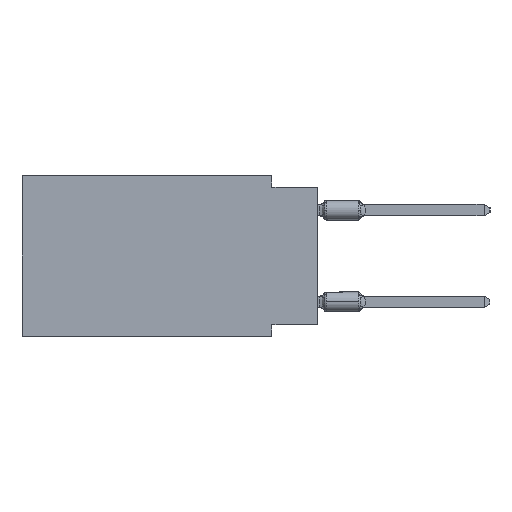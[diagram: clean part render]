
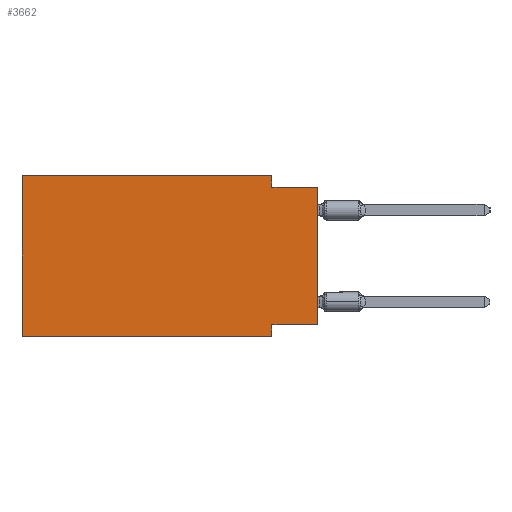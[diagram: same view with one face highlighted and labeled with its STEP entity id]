
A CAD part, left-side view. The second image highlights one B-rep face of the part: STEP entity #3662.
In plain terms, the highlighted planar face has unit normal (-1, 0, 0).
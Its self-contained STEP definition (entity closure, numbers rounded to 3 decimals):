
#502 = ORIENTED_EDGE ( 'NONE', *, *, #22959, .F. ) ;
#1128 = VERTEX_POINT ( 'NONE', #4056 ) ;
#3191 = VERTEX_POINT ( 'NONE', #32529 ) ;
#3344 = ORIENTED_EDGE ( 'NONE', *, *, #11986, .F. ) ;
#3662 = ADVANCED_FACE ( 'NONE', ( #44472 ), #28444, .F. ) ;
#3699 = EDGE_CURVE ( 'NONE', #20973, #11544, #36913, .T. ) ;
#3856 = ORIENTED_EDGE ( 'NONE', *, *, #19612, .F. ) ;
#4056 = CARTESIAN_POINT ( 'NONE',  ( 0., 16.383, 0. ) ) ;
#4516 = LINE ( 'NONE', #12303, #45934 ) ;
#4720 = CARTESIAN_POINT ( 'NONE',  ( 0., 16.383, 0. ) ) ;
#4727 = CARTESIAN_POINT ( 'NONE',  ( 0., 16.383, -8.89 ) ) ;
#4872 = EDGE_CURVE ( 'NONE', #45714, #3191, #16294, .T. ) ;
#4977 = CARTESIAN_POINT ( 'NONE',  ( 0., 2.54, -8.255 ) ) ;
#5626 = DIRECTION ( 'NONE',  ( 0., 0., 1. ) ) ;
#8097 = DIRECTION ( 'NONE',  ( 0., 1., 0. ) ) ;
#8184 = DIRECTION ( 'NONE',  ( 0., -1., 0. ) ) ;
#8557 = LINE ( 'NONE', #40531, #42065 ) ;
#8668 = CARTESIAN_POINT ( 'NONE',  ( 0., 16.383, 0. ) ) ;
#8676 = VECTOR ( 'NONE', #39610, 1000. ) ;
#8879 = CARTESIAN_POINT ( 'NONE',  ( 0., 0., -0.635 ) ) ;
#9559 = CARTESIAN_POINT ( 'NONE',  ( 0., 0., -8.255 ) ) ;
#11544 = VERTEX_POINT ( 'NONE', #21181 ) ;
#11986 = EDGE_CURVE ( 'NONE', #35517, #30591, #19890, .T. ) ;
#12303 = CARTESIAN_POINT ( 'NONE',  ( 0., 16.383, 0. ) ) ;
#12323 = CARTESIAN_POINT ( 'NONE',  ( 0., 16.383, -8.89 ) ) ;
#14198 = EDGE_CURVE ( 'NONE', #30591, #11544, #34202, .T. ) ;
#15579 = DIRECTION ( 'NONE',  ( 1., 0., 0. ) ) ;
#16291 = VECTOR ( 'NONE', #44668, 1000. ) ;
#16294 = LINE ( 'NONE', #4727, #21934 ) ;
#16332 = DIRECTION ( 'NONE',  ( 0., 0., -1. ) ) ;
#17349 = ORIENTED_EDGE ( 'NONE', *, *, #30152, .F. ) ;
#18081 = AXIS2_PLACEMENT_3D ( 'NONE', #4720, #15579, #32232 ) ;
#18759 = VERTEX_POINT ( 'NONE', #4977 ) ;
#19104 = LINE ( 'NONE', #8668, #16291 ) ;
#19604 = CARTESIAN_POINT ( 'NONE',  ( 0., 0., 0. ) ) ;
#19612 = EDGE_CURVE ( 'NONE', #1128, #35517, #4516, .T. ) ;
#19890 = LINE ( 'NONE', #24372, #28655 ) ;
#20842 = ORIENTED_EDGE ( 'NONE', *, *, #4872, .T. ) ;
#20973 = VERTEX_POINT ( 'NONE', #9559 ) ;
#21181 = CARTESIAN_POINT ( 'NONE',  ( 0., 0., -0.635 ) ) ;
#21934 = VECTOR ( 'NONE', #40700, 1000. ) ;
#22959 = EDGE_CURVE ( 'NONE', #18759, #3191, #43184, .T. ) ;
#24372 = CARTESIAN_POINT ( 'NONE',  ( 0., 2.54, 0. ) ) ;
#26332 = EDGE_LOOP ( 'NONE', ( #37521, #41750, #3344, #3856, #17349, #20842, #502, #34025 ) ) ;
#28444 = PLANE ( 'NONE',  #18081 ) ;
#28655 = VECTOR ( 'NONE', #16332, 1000. ) ;
#30152 = EDGE_CURVE ( 'NONE', #45714, #1128, #19104, .T. ) ;
#30591 = VERTEX_POINT ( 'NONE', #45070 ) ;
#31731 = EDGE_CURVE ( 'NONE', #20973, #18759, #8557, .T. ) ;
#32232 = DIRECTION ( 'NONE',  ( 0., 0., -1. ) ) ;
#32529 = CARTESIAN_POINT ( 'NONE',  ( 0., 2.54, -8.89 ) ) ;
#34025 = ORIENTED_EDGE ( 'NONE', *, *, #31731, .F. ) ;
#34202 = LINE ( 'NONE', #8879, #46009 ) ;
#35426 = VECTOR ( 'NONE', #5626, 1000. ) ;
#35517 = VERTEX_POINT ( 'NONE', #45631 ) ;
#36913 = LINE ( 'NONE', #19604, #35426 ) ;
#37521 = ORIENTED_EDGE ( 'NONE', *, *, #3699, .T. ) ;
#39610 = DIRECTION ( 'NONE',  ( 0., 0., -1. ) ) ;
#40531 = CARTESIAN_POINT ( 'NONE',  ( 0., 0., -8.255 ) ) ;
#40700 = DIRECTION ( 'NONE',  ( 0., -1., 0. ) ) ;
#41182 = DIRECTION ( 'NONE',  ( 0., -1., 0. ) ) ;
#41750 = ORIENTED_EDGE ( 'NONE', *, *, #14198, .F. ) ;
#42065 = VECTOR ( 'NONE', #8097, 1000. ) ;
#42944 = CARTESIAN_POINT ( 'NONE',  ( 0., 2.54, -8.89 ) ) ;
#43184 = LINE ( 'NONE', #42944, #8676 ) ;
#44472 = FACE_OUTER_BOUND ( 'NONE', #26332, .T. ) ;
#44668 = DIRECTION ( 'NONE',  ( 0., 0., 1. ) ) ;
#45070 = CARTESIAN_POINT ( 'NONE',  ( 0., 2.54, -0.635 ) ) ;
#45631 = CARTESIAN_POINT ( 'NONE',  ( 0., 2.54, 0. ) ) ;
#45714 = VERTEX_POINT ( 'NONE', #12323 ) ;
#45934 = VECTOR ( 'NONE', #41182, 1000. ) ;
#46009 = VECTOR ( 'NONE', #8184, 1000. ) ;
